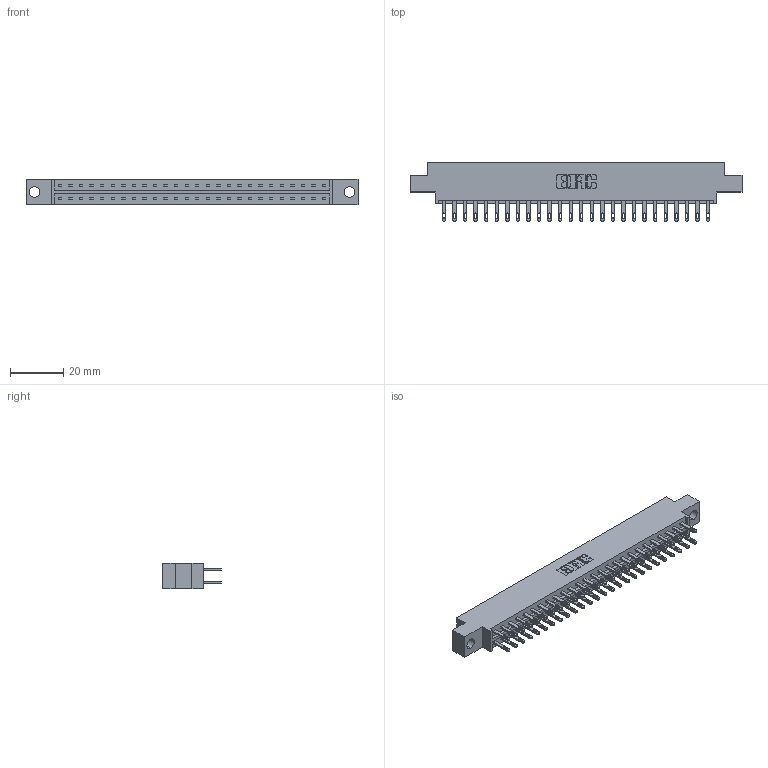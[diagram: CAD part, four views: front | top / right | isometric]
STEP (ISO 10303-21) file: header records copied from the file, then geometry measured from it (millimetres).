
FILE_DESCRIPTION (( 'STEP AP203' ), '1' );
FILE_NAME ('333-052-500-804.STEP', '2018-08-04T01:46:43', ( '' ), ( '' ), 'SwSTEP 2.0', 'SolidWorks 2016', '' );
FILE_SCHEMA (( 'CONFIG_CONTROL_DESIGN' ));
Length unit declared in the file: inch
Products named in the file (3): 333-052-500-804; 333 Part_Offset - .156 Dia - TH; 345-292-001_345-293-100
Assembly tree (53 placements, depth 2):
  333-052-500-804
    333 Part_Offset - .156 Dia - TH
    345-292-001_345-293-100  x52
Bounding box: 124.56 x 21.85 x 9.4 mm (x, y, z)
Volume: 12410.7 mm3; surface area: 15093 mm2
Topology: 53 solids, 53 shells, 2614 faces, 7967 edges, 5310 vertices
Faces by surface type: plane 1634, cylinder 980
Entity records: 18861 total; most frequent: CARTESIAN_POINT 3146, ORIENTED_EDGE 3082, DIRECTION 2717, EDGE_CURVE 1541, VECTOR 1409, LINE 1409, VERTEX_POINT 1026, AXIS2_PLACEMENT_3D 654
